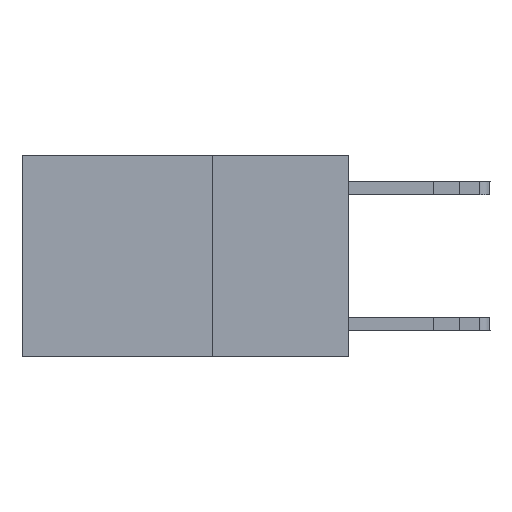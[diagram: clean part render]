
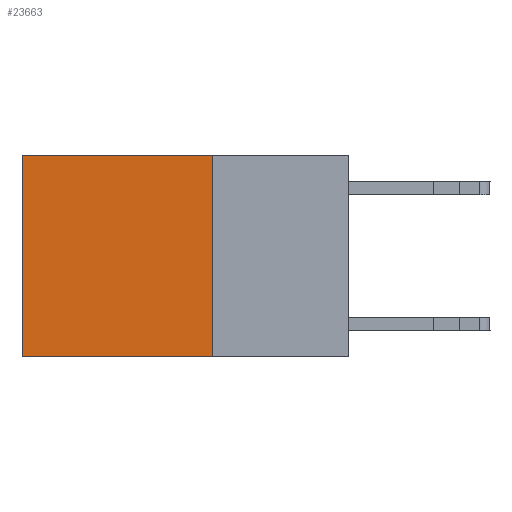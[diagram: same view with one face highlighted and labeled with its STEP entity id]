
A CAD part, left-side view. The second image highlights one B-rep face of the part: STEP entity #23663.
In plain terms, the highlighted planar face has unit normal (-1, 0, 0).
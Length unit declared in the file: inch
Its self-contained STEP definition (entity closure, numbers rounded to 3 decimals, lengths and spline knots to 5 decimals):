
#409 = LINE ( 'NONE', #541, #3012 ) ;
#418 = ORIENTED_EDGE ( 'NONE', *, *, #22259, .F. ) ;
#541 = CARTESIAN_POINT ( 'NONE',  ( 0.2625, 0.25, 0. ) ) ;
#1184 = ORIENTED_EDGE ( 'NONE', *, *, #21761, .T. ) ;
#3012 = VECTOR ( 'NONE', #15511, 39.37008 ) ;
#4374 = CARTESIAN_POINT ( 'NONE',  ( 0.2625, 0.6, 0. ) ) ;
#4470 = CARTESIAN_POINT ( 'NONE',  ( 0.2625, 0.25, 0. ) ) ;
#5140 = EDGE_CURVE ( 'NONE', #18410, #22512, #9062, .T. ) ;
#5538 = CARTESIAN_POINT ( 'NONE',  ( 0.2625, 0.25, 0. ) ) ;
#5553 = VERTEX_POINT ( 'NONE', #4374 ) ;
#6681 = EDGE_CURVE ( 'NONE', #17775, #5553, #409, .T. ) ;
#7394 = FACE_OUTER_BOUND ( 'NONE', #21678, .T. ) ;
#8622 = AXIS2_PLACEMENT_3D ( 'NONE', #5538, #9216, #16700 ) ;
#9062 = LINE ( 'NONE', #14579, #22413 ) ;
#9216 = DIRECTION ( 'NONE',  ( 1., 0., 0. ) ) ;
#10108 = ORIENTED_EDGE ( 'NONE', *, *, #6681, .T. ) ;
#10745 = CARTESIAN_POINT ( 'NONE',  ( 0.2625, 0.25, 0. ) ) ;
#11692 = DIRECTION ( 'NONE',  ( 0., 0., -1. ) ) ;
#13421 = LINE ( 'NONE', #19158, #23721 ) ;
#14579 = CARTESIAN_POINT ( 'NONE',  ( 0.2625, 0.25, -0.37 ) ) ;
#15511 = DIRECTION ( 'NONE',  ( 0., 1., 0. ) ) ;
#16700 = DIRECTION ( 'NONE',  ( 0., 0., -1. ) ) ;
#16896 = DIRECTION ( 'NONE',  ( 0., 1., 0. ) ) ;
#17775 = VERTEX_POINT ( 'NONE', #10745 ) ;
#18410 = VERTEX_POINT ( 'NONE', #19922 ) ;
#18511 = PLANE ( 'NONE',  #8622 ) ;
#19158 = CARTESIAN_POINT ( 'NONE',  ( 0.2625, 0.6, 0. ) ) ;
#19389 = DIRECTION ( 'NONE',  ( 0., 0., -1. ) ) ;
#19922 = CARTESIAN_POINT ( 'NONE',  ( 0.2625, 0.25, -0.37 ) ) ;
#20441 = CARTESIAN_POINT ( 'NONE',  ( 0.2625, 0.6, -0.37 ) ) ;
#21678 = EDGE_LOOP ( 'NONE', ( #1184, #23502, #418, #10108 ) ) ;
#21761 = EDGE_CURVE ( 'NONE', #5553, #22512, #13421, .T. ) ;
#22259 = EDGE_CURVE ( 'NONE', #17775, #18410, #23039, .T. ) ;
#22413 = VECTOR ( 'NONE', #16896, 39.37008 ) ;
#22512 = VERTEX_POINT ( 'NONE', #20441 ) ;
#22562 = VECTOR ( 'NONE', #11692, 39.37008 ) ;
#23039 = LINE ( 'NONE', #4470, #22562 ) ;
#23502 = ORIENTED_EDGE ( 'NONE', *, *, #5140, .F. ) ;
#23663 = ADVANCED_FACE ( 'NONE', ( #7394 ), #18511, .F. ) ;
#23721 = VECTOR ( 'NONE', #19389, 39.37008 ) ;
